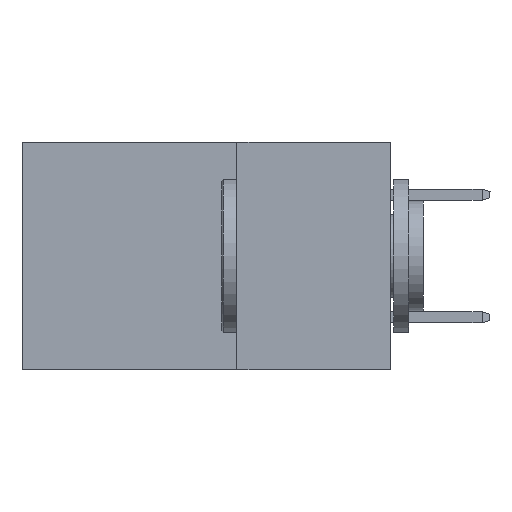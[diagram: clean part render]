
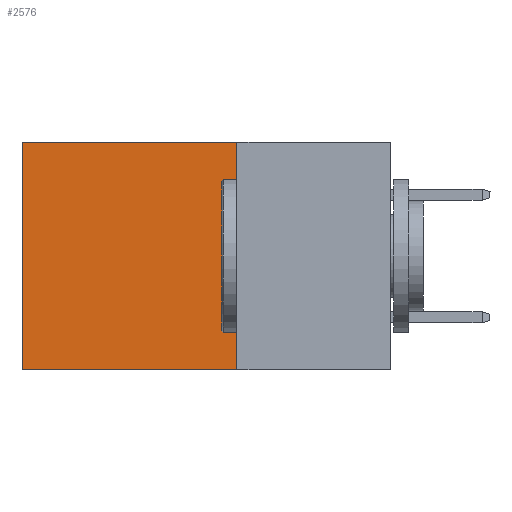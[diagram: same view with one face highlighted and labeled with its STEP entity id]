
A CAD part, left-side view. The second image highlights one B-rep face of the part: STEP entity #2576.
In plain terms, the highlighted planar face has unit normal (-1, 0, 0).
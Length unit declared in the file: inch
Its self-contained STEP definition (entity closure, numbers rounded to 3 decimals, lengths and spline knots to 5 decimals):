
#463 = DIRECTION ( 'NONE',  ( 0., 0., -1. ) ) ;
#2576 = ADVANCED_FACE ( 'NONE', ( #42020 ), #41395, .F. ) ;
#3293 = LINE ( 'NONE', #36704, #11766 ) ;
#4364 = ORIENTED_EDGE ( 'NONE', *, *, #13208, .T. ) ;
#9857 = VECTOR ( 'NONE', #43092, 39.37008 ) ;
#11239 = CARTESIAN_POINT ( 'NONE',  ( 0.2875, 0.6, 0. ) ) ;
#11500 = VERTEX_POINT ( 'NONE', #41932 ) ;
#11766 = VECTOR ( 'NONE', #463, 39.37008 ) ;
#12389 = EDGE_CURVE ( 'NONE', #15118, #11500, #21817, .T. ) ;
#13208 = EDGE_CURVE ( 'NONE', #44182, #11500, #44252, .T. ) ;
#14117 = AXIS2_PLACEMENT_3D ( 'NONE', #37780, #44925, #23392 ) ;
#14512 = EDGE_CURVE ( 'NONE', #39788, #15118, #3293, .T. ) ;
#14962 = ORIENTED_EDGE ( 'NONE', *, *, #45421, .T. ) ;
#15118 = VERTEX_POINT ( 'NONE', #21596 ) ;
#17885 = ORIENTED_EDGE ( 'NONE', *, *, #14512, .F. ) ;
#19860 = LINE ( 'NONE', #46527, #29490 ) ;
#20893 = ORIENTED_EDGE ( 'NONE', *, *, #12389, .F. ) ;
#21596 = CARTESIAN_POINT ( 'NONE',  ( 0.2875, 0.25, -0.37 ) ) ;
#21817 = LINE ( 'NONE', #39364, #9857 ) ;
#22061 = DIRECTION ( 'NONE',  ( 0., 0., -1. ) ) ;
#23392 = DIRECTION ( 'NONE',  ( 0., 0., -1. ) ) ;
#29490 = VECTOR ( 'NONE', #39407, 39.37008 ) ;
#31059 = EDGE_LOOP ( 'NONE', ( #4364, #20893, #17885, #14962 ) ) ;
#32466 = VECTOR ( 'NONE', #22061, 39.37008 ) ;
#36704 = CARTESIAN_POINT ( 'NONE',  ( 0.2875, 0.25, 0. ) ) ;
#37780 = CARTESIAN_POINT ( 'NONE',  ( 0.2875, 0.25, 0. ) ) ;
#39364 = CARTESIAN_POINT ( 'NONE',  ( 0.2875, 0.25, -0.37 ) ) ;
#39407 = DIRECTION ( 'NONE',  ( 0., 1., 0. ) ) ;
#39788 = VERTEX_POINT ( 'NONE', #41831 ) ;
#41395 = PLANE ( 'NONE',  #14117 ) ;
#41831 = CARTESIAN_POINT ( 'NONE',  ( 0.2875, 0.25, 0. ) ) ;
#41932 = CARTESIAN_POINT ( 'NONE',  ( 0.2875, 0.6, -0.37 ) ) ;
#42014 = CARTESIAN_POINT ( 'NONE',  ( 0.2875, 0.6, 0. ) ) ;
#42020 = FACE_OUTER_BOUND ( 'NONE', #31059, .T. ) ;
#43092 = DIRECTION ( 'NONE',  ( 0., 1., 0. ) ) ;
#44182 = VERTEX_POINT ( 'NONE', #42014 ) ;
#44252 = LINE ( 'NONE', #11239, #32466 ) ;
#44925 = DIRECTION ( 'NONE',  ( 1., 0., 0. ) ) ;
#45421 = EDGE_CURVE ( 'NONE', #39788, #44182, #19860, .T. ) ;
#46527 = CARTESIAN_POINT ( 'NONE',  ( 0.2875, 0.25, 0. ) ) ;
